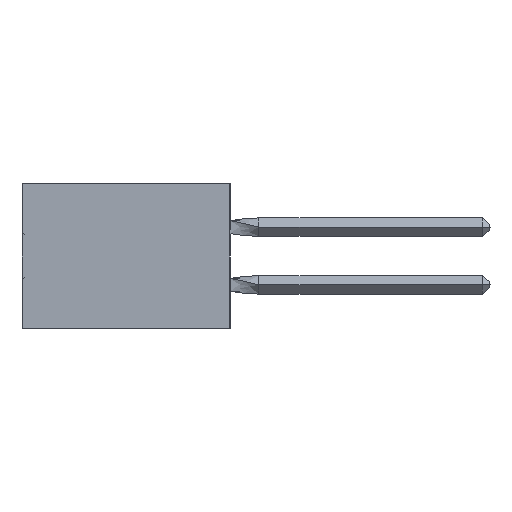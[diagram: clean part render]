
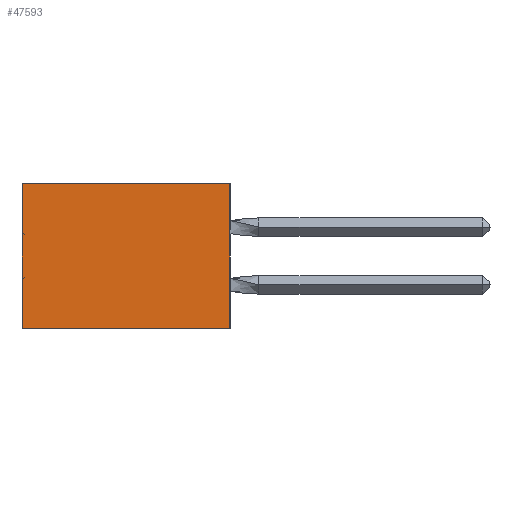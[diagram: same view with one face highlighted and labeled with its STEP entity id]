
A CAD part, left-side view. The second image highlights one B-rep face of the part: STEP entity #47593.
In plain terms, the highlighted planar face has unit normal (-1, 0, 0).
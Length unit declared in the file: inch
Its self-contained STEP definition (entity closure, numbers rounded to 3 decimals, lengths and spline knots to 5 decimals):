
#111 = LINE ( 'NONE', #40055, #31380 ) ;
#698 = LINE ( 'NONE', #34488, #10368 ) ;
#5276 = VECTOR ( 'NONE', #20759, 39.37008 ) ;
#5965 = DIRECTION ( 'NONE',  ( 0., 0., -1. ) ) ;
#6445 = DIRECTION ( 'NONE',  ( 0., 0., -1. ) ) ;
#6834 = VERTEX_POINT ( 'NONE', #13603 ) ;
#8640 = ORIENTED_EDGE ( 'NONE', *, *, #41844, .F. ) ;
#10368 = VECTOR ( 'NONE', #5965, 39.37008 ) ;
#10846 = PLANE ( 'NONE',  #46595 ) ;
#11231 = CARTESIAN_POINT ( 'NONE',  ( 0.305, 0., -0.5 ) ) ;
#13603 = CARTESIAN_POINT ( 'NONE',  ( 0.305, 0., 0. ) ) ;
#15361 = EDGE_LOOP ( 'NONE', ( #22770, #8640, #50479, #24853 ) ) ;
#15989 = CARTESIAN_POINT ( 'NONE',  ( 0.305, 0., -0.5 ) ) ;
#17269 = VECTOR ( 'NONE', #29856, 39.37008 ) ;
#17949 = LINE ( 'NONE', #15989, #5276 ) ;
#20454 = VERTEX_POINT ( 'NONE', #56674 ) ;
#20759 = DIRECTION ( 'NONE',  ( 0., 0., -1. ) ) ;
#22770 = ORIENTED_EDGE ( 'NONE', *, *, #43726, .T. ) ;
#24853 = ORIENTED_EDGE ( 'NONE', *, *, #30858, .T. ) ;
#29439 = CARTESIAN_POINT ( 'NONE',  ( 0.305, 0., 0. ) ) ;
#29856 = DIRECTION ( 'NONE',  ( 0., 1., 0. ) ) ;
#30858 = EDGE_CURVE ( 'NONE', #6834, #53564, #44074, .T. ) ;
#31380 = VECTOR ( 'NONE', #58790, 39.37008 ) ;
#34488 = CARTESIAN_POINT ( 'NONE',  ( 0.305, 0.72, -0.5 ) ) ;
#39436 = EDGE_CURVE ( 'NONE', #6834, #40804, #17949, .T. ) ;
#39745 = CARTESIAN_POINT ( 'NONE',  ( 0.305, 0., -0.5 ) ) ;
#40055 = CARTESIAN_POINT ( 'NONE',  ( 0.305, 0., -0.5 ) ) ;
#40501 = CARTESIAN_POINT ( 'NONE',  ( 0.305, 0.72, 0. ) ) ;
#40804 = VERTEX_POINT ( 'NONE', #39745 ) ;
#41844 = EDGE_CURVE ( 'NONE', #40804, #20454, #111, .T. ) ;
#43726 = EDGE_CURVE ( 'NONE', #53564, #20454, #698, .T. ) ;
#44074 = LINE ( 'NONE', #29439, #17269 ) ;
#44087 = DIRECTION ( 'NONE',  ( 1., 0., 0. ) ) ;
#46595 = AXIS2_PLACEMENT_3D ( 'NONE', #11231, #44087, #6445 ) ;
#47593 = ADVANCED_FACE ( 'NONE', ( #50765 ), #10846, .F. ) ;
#50479 = ORIENTED_EDGE ( 'NONE', *, *, #39436, .F. ) ;
#50765 = FACE_OUTER_BOUND ( 'NONE', #15361, .T. ) ;
#53564 = VERTEX_POINT ( 'NONE', #40501 ) ;
#56674 = CARTESIAN_POINT ( 'NONE',  ( 0.305, 0.72, -0.5 ) ) ;
#58790 = DIRECTION ( 'NONE',  ( 0., 1., 0. ) ) ;
